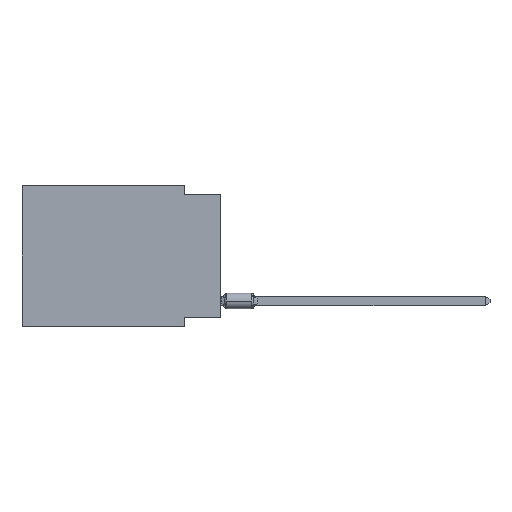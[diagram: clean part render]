
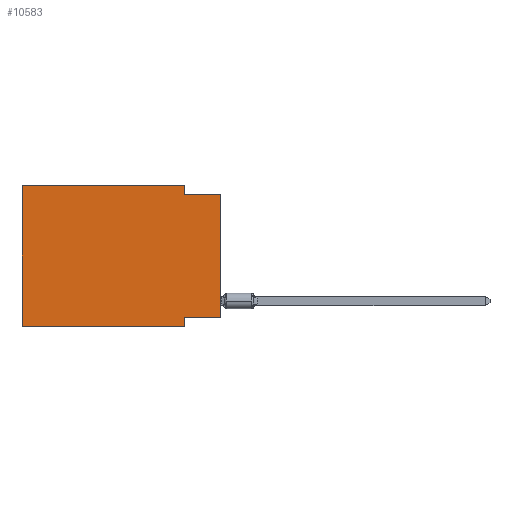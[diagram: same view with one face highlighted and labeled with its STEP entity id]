
A CAD part, left-side view. The second image highlights one B-rep face of the part: STEP entity #10583.
In plain terms, the highlighted planar face has unit normal (-1, 0, 0).
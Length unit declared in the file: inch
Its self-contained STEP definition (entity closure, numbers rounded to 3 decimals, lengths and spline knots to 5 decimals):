
#244 = ORIENTED_EDGE ( 'NONE', *, *, #7324, .F. ) ;
#379 = CARTESIAN_POINT ( 'NONE',  ( 0., 0.1, -0.39 ) ) ;
#412 = CARTESIAN_POINT ( 'NONE',  ( 0., 0.55, -0.39 ) ) ;
#473 = VERTEX_POINT ( 'NONE', #412 ) ;
#528 = CARTESIAN_POINT ( 'NONE',  ( 0., 0.55, -0.39 ) ) ;
#818 = EDGE_CURVE ( 'NONE', #12360, #8955, #13656, .T. ) ;
#952 = CARTESIAN_POINT ( 'NONE',  ( 0., 0.55, 0. ) ) ;
#1042 = EDGE_CURVE ( 'NONE', #473, #4267, #3171, .T. ) ;
#1084 = VECTOR ( 'NONE', #7674, 39.37008 ) ;
#1446 = CARTESIAN_POINT ( 'NONE',  ( 0., 0.1, -0.365 ) ) ;
#1513 = CARTESIAN_POINT ( 'NONE',  ( 0., 0.1, -0.025 ) ) ;
#2153 = ORIENTED_EDGE ( 'NONE', *, *, #5074, .T. ) ;
#2247 = DIRECTION ( 'NONE',  ( 1., 0., 0. ) ) ;
#2467 = VERTEX_POINT ( 'NONE', #379 ) ;
#2748 = AXIS2_PLACEMENT_3D ( 'NONE', #4886, #2247, #11154 ) ;
#2753 = CARTESIAN_POINT ( 'NONE',  ( 0., 0.55, 0. ) ) ;
#3117 = EDGE_CURVE ( 'NONE', #13330, #12360, #4450, .T. ) ;
#3171 = LINE ( 'NONE', #7549, #12969 ) ;
#4024 = VERTEX_POINT ( 'NONE', #1446 ) ;
#4267 = VERTEX_POINT ( 'NONE', #952 ) ;
#4450 = LINE ( 'NONE', #7742, #1084 ) ;
#4534 = CARTESIAN_POINT ( 'NONE',  ( 0., 0.1, 0. ) ) ;
#4886 = CARTESIAN_POINT ( 'NONE',  ( 0., 0.55, 0. ) ) ;
#4902 = DIRECTION ( 'NONE',  ( 0., -1., 0. ) ) ;
#4956 = DIRECTION ( 'NONE',  ( 0., 1., 0. ) ) ;
#5074 = EDGE_CURVE ( 'NONE', #10532, #8955, #8360, .T. ) ;
#5196 = ORIENTED_EDGE ( 'NONE', *, *, #1042, .F. ) ;
#5372 = VECTOR ( 'NONE', #8128, 39.37008 ) ;
#5390 = EDGE_CURVE ( 'NONE', #4267, #13330, #5990, .T. ) ;
#5422 = ORIENTED_EDGE ( 'NONE', *, *, #3117, .F. ) ;
#5820 = LINE ( 'NONE', #10203, #13531 ) ;
#5824 = LINE ( 'NONE', #6972, #6909 ) ;
#5990 = LINE ( 'NONE', #2753, #13118 ) ;
#6190 = LINE ( 'NONE', #528, #7813 ) ;
#6784 = EDGE_CURVE ( 'NONE', #10532, #4024, #5820, .T. ) ;
#6849 = DIRECTION ( 'NONE',  ( 0., -1., 0. ) ) ;
#6909 = VECTOR ( 'NONE', #12649, 39.37008 ) ;
#6912 = CARTESIAN_POINT ( 'NONE',  ( 0., 0., -0.025 ) ) ;
#6972 = CARTESIAN_POINT ( 'NONE',  ( 0., 0.1, -0.39 ) ) ;
#7285 = CARTESIAN_POINT ( 'NONE',  ( 0., 0., -0.365 ) ) ;
#7324 = EDGE_CURVE ( 'NONE', #4024, #2467, #5824, .T. ) ;
#7549 = CARTESIAN_POINT ( 'NONE',  ( 0., 0.55, 0. ) ) ;
#7674 = DIRECTION ( 'NONE',  ( 0., 0., -1. ) ) ;
#7742 = CARTESIAN_POINT ( 'NONE',  ( 0., 0.1, 0. ) ) ;
#7813 = VECTOR ( 'NONE', #4902, 39.37008 ) ;
#8128 = DIRECTION ( 'NONE',  ( 0., -1., 0. ) ) ;
#8232 = ORIENTED_EDGE ( 'NONE', *, *, #818, .F. ) ;
#8360 = LINE ( 'NONE', #12826, #9500 ) ;
#8955 = VERTEX_POINT ( 'NONE', #13836 ) ;
#9500 = VECTOR ( 'NONE', #11674, 39.37008 ) ;
#9945 = ORIENTED_EDGE ( 'NONE', *, *, #6784, .F. ) ;
#9995 = PLANE ( 'NONE',  #2748 ) ;
#10203 = CARTESIAN_POINT ( 'NONE',  ( 0., 0., -0.365 ) ) ;
#10532 = VERTEX_POINT ( 'NONE', #7285 ) ;
#10567 = ORIENTED_EDGE ( 'NONE', *, *, #5390, .F. ) ;
#10583 = ADVANCED_FACE ( 'NONE', ( #12295 ), #9995, .F. ) ;
#11154 = DIRECTION ( 'NONE',  ( 0., 0., -1. ) ) ;
#11175 = ORIENTED_EDGE ( 'NONE', *, *, #11865, .T. ) ;
#11674 = DIRECTION ( 'NONE',  ( 0., 0., 1. ) ) ;
#11865 = EDGE_CURVE ( 'NONE', #473, #2467, #6190, .T. ) ;
#11939 = DIRECTION ( 'NONE',  ( 0., 0., 1. ) ) ;
#12295 = FACE_OUTER_BOUND ( 'NONE', #14091, .T. ) ;
#12360 = VERTEX_POINT ( 'NONE', #1513 ) ;
#12649 = DIRECTION ( 'NONE',  ( 0., 0., -1. ) ) ;
#12826 = CARTESIAN_POINT ( 'NONE',  ( 0., 0., 0. ) ) ;
#12969 = VECTOR ( 'NONE', #11939, 39.37008 ) ;
#13118 = VECTOR ( 'NONE', #6849, 39.37008 ) ;
#13330 = VERTEX_POINT ( 'NONE', #4534 ) ;
#13531 = VECTOR ( 'NONE', #4956, 39.37008 ) ;
#13656 = LINE ( 'NONE', #6912, #5372 ) ;
#13836 = CARTESIAN_POINT ( 'NONE',  ( 0., 0., -0.025 ) ) ;
#14091 = EDGE_LOOP ( 'NONE', ( #2153, #8232, #5422, #10567, #5196, #11175, #244, #9945 ) ) ;
